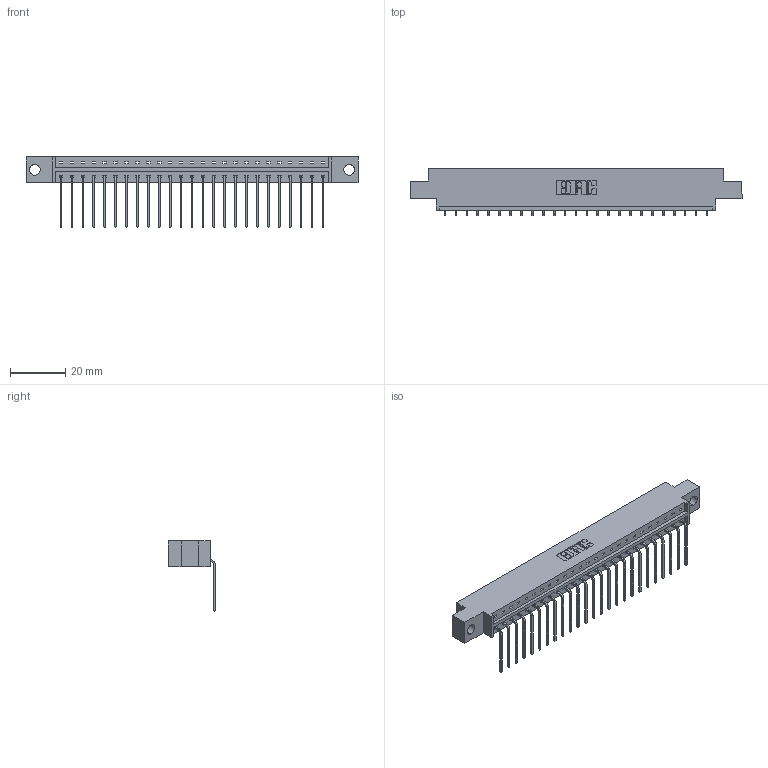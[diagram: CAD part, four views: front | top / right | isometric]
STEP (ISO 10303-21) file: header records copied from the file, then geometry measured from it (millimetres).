
FILE_DESCRIPTION (( 'STEP AP203' ), '1' );
FILE_NAME ('333-025-559-604.STEP', '2018-08-02T12:21:21', ( '' ), ( '' ), 'SwSTEP 2.0', 'SolidWorks 2016', '' );
FILE_SCHEMA (( 'CONFIG_CONTROL_DESIGN' ));
Length unit declared in the file: inch
Products named in the file (3): 345-292-001_558 559 Tail - 1; 333-025-559-604; 333 Part_Offset - .156 Dia - TH
Assembly tree (26 placements, depth 2):
  333-025-559-604
    333 Part_Offset - .156 Dia - TH
    345-292-001_558 559 Tail - 1  x25
Bounding box: 120.6 x 17.09 x 25.53 mm (x, y, z)
Volume: 11757.1 mm3; surface area: 13113.9 mm2
Topology: 26 solids, 26 shells, 1618 faces, 4873 edges, 3214 vertices
Faces by surface type: plane 1174, cylinder 444
Entity records: 17701 total; most frequent: CARTESIAN_POINT 3065, ORIENTED_EDGE 3026, DIRECTION 2619, EDGE_CURVE 1513, LINE 1385, VECTOR 1385, VERTEX_POINT 1006, AXIS2_PLACEMENT_3D 617
